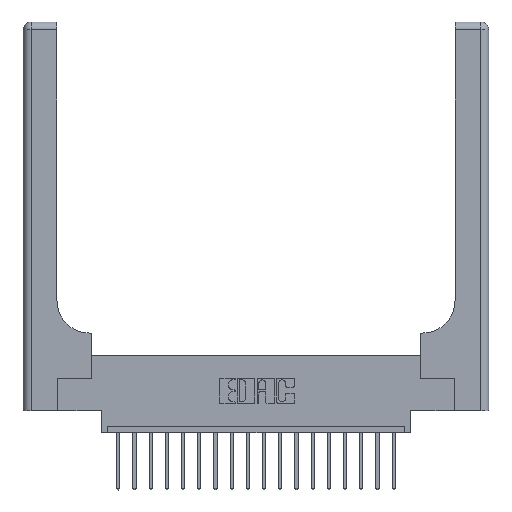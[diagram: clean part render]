
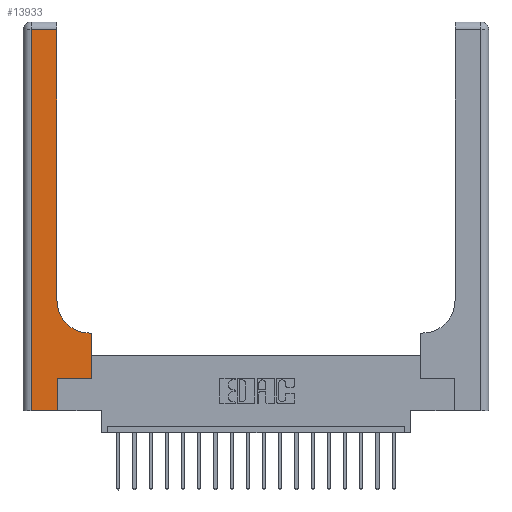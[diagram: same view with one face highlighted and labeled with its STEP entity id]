
A CAD part, top view. The second image highlights one B-rep face of the part: STEP entity #13933.
In plain terms, the highlighted planar face has unit normal (0, 0, 1).
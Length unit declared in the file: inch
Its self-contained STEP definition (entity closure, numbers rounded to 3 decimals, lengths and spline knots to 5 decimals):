
#46 = LINE ( 'NONE', #12334, #11770 ) ;
#279 = DIRECTION ( 'NONE',  ( -1., 0., 0. ) ) ;
#413 = LINE ( 'NONE', #3792, #2807 ) ;
#463 = DIRECTION ( 'NONE',  ( 1., 0., 0. ) ) ;
#1394 = ORIENTED_EDGE ( 'NONE', *, *, #6793, .T. ) ;
#1460 = VECTOR ( 'NONE', #9638, 39.37008 ) ;
#1516 = AXIS2_PLACEMENT_3D ( 'NONE', #16993, #9372, #463 ) ;
#1545 = ORIENTED_EDGE ( 'NONE', *, *, #16132, .T. ) ;
#1614 = DIRECTION ( 'NONE',  ( 0., 0., -1. ) ) ;
#1699 = LINE ( 'NONE', #6683, #2655 ) ;
#1781 = CARTESIAN_POINT ( 'NONE',  ( 0.51, 0.6, 0.37 ) ) ;
#2386 = EDGE_CURVE ( 'NONE', #17073, #4727, #46, .T. ) ;
#2655 = VECTOR ( 'NONE', #3807, 39.37008 ) ;
#2807 = VECTOR ( 'NONE', #17642, 39.37008 ) ;
#2830 = LINE ( 'NONE', #10660, #7074 ) ;
#2992 = EDGE_CURVE ( 'NONE', #4727, #3095, #15556, .T. ) ;
#3085 = CARTESIAN_POINT ( 'NONE',  ( 0., 3., 0.37 ) ) ;
#3095 = VERTEX_POINT ( 'NONE', #1781 ) ;
#3202 = EDGE_CURVE ( 'NONE', #15810, #17193, #413, .T. ) ;
#3792 = CARTESIAN_POINT ( 'NONE',  ( 0., 2.94, 0.37 ) ) ;
#3807 = DIRECTION ( 'NONE',  ( 0., 1., 0. ) ) ;
#4072 = LINE ( 'NONE', #17944, #12975 ) ;
#4727 = VERTEX_POINT ( 'NONE', #12156 ) ;
#5201 = CARTESIAN_POINT ( 'NONE',  ( 0.26, 0.85, 0.37 ) ) ;
#5207 = CARTESIAN_POINT ( 'NONE',  ( 0.26, 2.94, 0.37 ) ) ;
#5356 = FACE_OUTER_BOUND ( 'NONE', #16150, .T. ) ;
#5592 = DIRECTION ( 'NONE',  ( 1., 0., 0. ) ) ;
#5941 = CARTESIAN_POINT ( 'NONE',  ( 0.26, 0.6, 0.37 ) ) ;
#6064 = EDGE_CURVE ( 'NONE', #11766, #7231, #2830, .T. ) ;
#6540 = AXIS2_PLACEMENT_3D ( 'NONE', #3085, #1614, #279 ) ;
#6683 = CARTESIAN_POINT ( 'NONE',  ( 0.26, 3., 0.37 ) ) ;
#6793 = EDGE_CURVE ( 'NONE', #15392, #15810, #1699, .T. ) ;
#7074 = VECTOR ( 'NONE', #13845, 39.37008 ) ;
#7087 = LINE ( 'NONE', #15483, #18626 ) ;
#7231 = VERTEX_POINT ( 'NONE', #19026 ) ;
#7267 = DIRECTION ( 'NONE',  ( -1., 0., 0. ) ) ;
#8241 = DIRECTION ( 'NONE',  ( 0., 1., 0. ) ) ;
#9372 = DIRECTION ( 'NONE',  ( 0., 0., -1. ) ) ;
#9638 = DIRECTION ( 'NONE',  ( 1., 0., 0. ) ) ;
#9937 = CARTESIAN_POINT ( 'NONE',  ( 0.06, 0., 0.37 ) ) ;
#10508 = ORIENTED_EDGE ( 'NONE', *, *, #6064, .T. ) ;
#10595 = EDGE_CURVE ( 'NONE', #12112, #11766, #13499, .T. ) ;
#10660 = CARTESIAN_POINT ( 'NONE',  ( 0.265, 0., 0.37 ) ) ;
#10936 = VECTOR ( 'NONE', #7267, 39.37008 ) ;
#11188 = CARTESIAN_POINT ( 'NONE',  ( 0.528, 0.25, 0.37 ) ) ;
#11680 = EDGE_CURVE ( 'NONE', #7231, #17073, #4072, .T. ) ;
#11766 = VERTEX_POINT ( 'NONE', #13602 ) ;
#11770 = VECTOR ( 'NONE', #8241, 39.37008 ) ;
#12004 = EDGE_CURVE ( 'NONE', #17193, #12112, #7087, .T. ) ;
#12112 = VERTEX_POINT ( 'NONE', #9937 ) ;
#12156 = CARTESIAN_POINT ( 'NONE',  ( 0.528, 0.6, 0.37 ) ) ;
#12180 = ORIENTED_EDGE ( 'NONE', *, *, #2992, .T. ) ;
#12334 = CARTESIAN_POINT ( 'NONE',  ( 0.528, 0.25, 0.37 ) ) ;
#12624 = CARTESIAN_POINT ( 'NONE',  ( 0., 0., 0.37 ) ) ;
#12975 = VECTOR ( 'NONE', #5592, 39.37008 ) ;
#13499 = LINE ( 'NONE', #12624, #1460 ) ;
#13602 = CARTESIAN_POINT ( 'NONE',  ( 0.265, 0., 0.37 ) ) ;
#13757 = ORIENTED_EDGE ( 'NONE', *, *, #12004, .T. ) ;
#13845 = DIRECTION ( 'NONE',  ( 0., 1., 0. ) ) ;
#13933 = ADVANCED_FACE ( 'NONE', ( #5356 ), #17134, .F. ) ;
#15392 = VERTEX_POINT ( 'NONE', #5201 ) ;
#15483 = CARTESIAN_POINT ( 'NONE',  ( 0.06, 3., 0.37 ) ) ;
#15556 = LINE ( 'NONE', #5941, #10936 ) ;
#15810 = VERTEX_POINT ( 'NONE', #5207 ) ;
#15924 = CIRCLE ( 'NONE', #1516, 0.25 ) ;
#16132 = EDGE_CURVE ( 'NONE', #3095, #15392, #15924, .T. ) ;
#16150 = EDGE_LOOP ( 'NONE', ( #1394, #17329, #13757, #18454, #10508, #18697, #18497, #12180, #1545 ) ) ;
#16993 = CARTESIAN_POINT ( 'NONE',  ( 0.51, 0.85, 0.37 ) ) ;
#17073 = VERTEX_POINT ( 'NONE', #11188 ) ;
#17134 = PLANE ( 'NONE',  #6540 ) ;
#17193 = VERTEX_POINT ( 'NONE', #18688 ) ;
#17329 = ORIENTED_EDGE ( 'NONE', *, *, #3202, .T. ) ;
#17521 = DIRECTION ( 'NONE',  ( 0., -1., 0. ) ) ;
#17642 = DIRECTION ( 'NONE',  ( -1., 0., 0. ) ) ;
#17944 = CARTESIAN_POINT ( 'NONE',  ( 0.265, 0.25, 0.37 ) ) ;
#18454 = ORIENTED_EDGE ( 'NONE', *, *, #10595, .T. ) ;
#18497 = ORIENTED_EDGE ( 'NONE', *, *, #2386, .T. ) ;
#18626 = VECTOR ( 'NONE', #17521, 39.37008 ) ;
#18688 = CARTESIAN_POINT ( 'NONE',  ( 0.06, 2.94, 0.37 ) ) ;
#18697 = ORIENTED_EDGE ( 'NONE', *, *, #11680, .T. ) ;
#19026 = CARTESIAN_POINT ( 'NONE',  ( 0.265, 0.25, 0.37 ) ) ;
